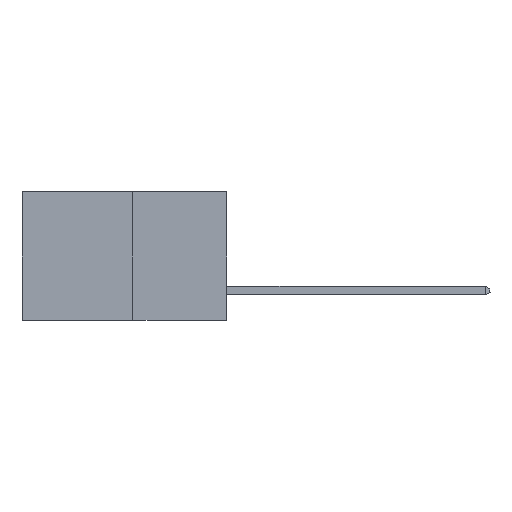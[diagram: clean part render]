
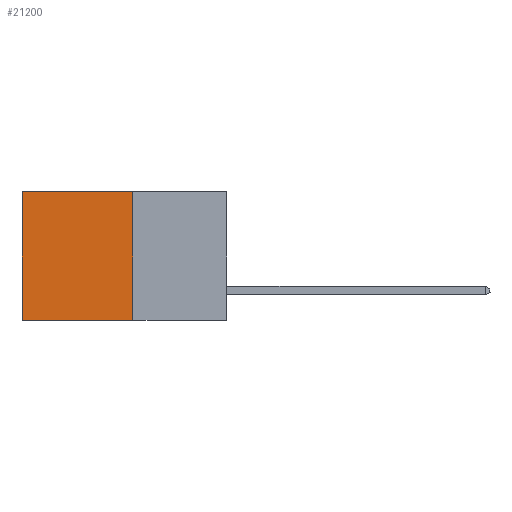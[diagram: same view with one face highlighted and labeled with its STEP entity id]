
A CAD part, left-side view. The second image highlights one B-rep face of the part: STEP entity #21200.
In plain terms, the highlighted planar face has unit normal (-1, 0, 0).
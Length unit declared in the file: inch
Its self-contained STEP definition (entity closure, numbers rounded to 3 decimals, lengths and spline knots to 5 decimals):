
#597 = EDGE_CURVE ( 'NONE', #8936, #16525, #10920, .T. ) ;
#1266 = CARTESIAN_POINT ( 'NONE',  ( 0.277, 0.27, 0. ) ) ;
#1617 = ORIENTED_EDGE ( 'NONE', *, *, #21291, .T. ) ;
#2578 = EDGE_LOOP ( 'NONE', ( #8515, #19043, #21522, #1617 ) ) ;
#2692 = PLANE ( 'NONE',  #3123 ) ;
#2982 = CARTESIAN_POINT ( 'NONE',  ( 0.277, 0.27, 0. ) ) ;
#3123 = AXIS2_PLACEMENT_3D ( 'NONE', #6140, #7850, #19578 ) ;
#4445 = LINE ( 'NONE', #12794, #17361 ) ;
#5025 = VECTOR ( 'NONE', #19873, 39.37008 ) ;
#6140 = CARTESIAN_POINT ( 'NONE',  ( 0.277, 0.27, -0.37 ) ) ;
#6187 = CARTESIAN_POINT ( 'NONE',  ( 0.277, 0.59, 0. ) ) ;
#6732 = LINE ( 'NONE', #14711, #15118 ) ;
#7850 = DIRECTION ( 'NONE',  ( 1., 0., 0. ) ) ;
#7950 = CARTESIAN_POINT ( 'NONE',  ( 0.277, 0.27, -0.37 ) ) ;
#8515 = ORIENTED_EDGE ( 'NONE', *, *, #15218, .T. ) ;
#8936 = VERTEX_POINT ( 'NONE', #7950 ) ;
#9495 = LINE ( 'NONE', #2982, #5025 ) ;
#10231 = CARTESIAN_POINT ( 'NONE',  ( 0.277, 0.59, -0.37 ) ) ;
#10920 = LINE ( 'NONE', #15836, #19350 ) ;
#11123 = VERTEX_POINT ( 'NONE', #1266 ) ;
#12794 = CARTESIAN_POINT ( 'NONE',  ( 0.277, 0.59, -0.37 ) ) ;
#13397 = EDGE_CURVE ( 'NONE', #11123, #8936, #6732, .T. ) ;
#14039 = VERTEX_POINT ( 'NONE', #6187 ) ;
#14504 = DIRECTION ( 'NONE',  ( 0., 0., -1. ) ) ;
#14711 = CARTESIAN_POINT ( 'NONE',  ( 0.277, 0.27, -0.37 ) ) ;
#14786 = DIRECTION ( 'NONE',  ( 0., 0., -1. ) ) ;
#15118 = VECTOR ( 'NONE', #14786, 39.37008 ) ;
#15218 = EDGE_CURVE ( 'NONE', #14039, #16525, #4445, .T. ) ;
#15836 = CARTESIAN_POINT ( 'NONE',  ( 0.277, 0.27, -0.37 ) ) ;
#16525 = VERTEX_POINT ( 'NONE', #10231 ) ;
#17361 = VECTOR ( 'NONE', #14504, 39.37008 ) ;
#19043 = ORIENTED_EDGE ( 'NONE', *, *, #597, .F. ) ;
#19350 = VECTOR ( 'NONE', #21571, 39.37008 ) ;
#19578 = DIRECTION ( 'NONE',  ( 0., 0., -1. ) ) ;
#19873 = DIRECTION ( 'NONE',  ( 0., 1., 0. ) ) ;
#21058 = FACE_OUTER_BOUND ( 'NONE', #2578, .T. ) ;
#21200 = ADVANCED_FACE ( 'NONE', ( #21058 ), #2692, .F. ) ;
#21291 = EDGE_CURVE ( 'NONE', #11123, #14039, #9495, .T. ) ;
#21522 = ORIENTED_EDGE ( 'NONE', *, *, #13397, .F. ) ;
#21571 = DIRECTION ( 'NONE',  ( 0., 1., 0. ) ) ;
